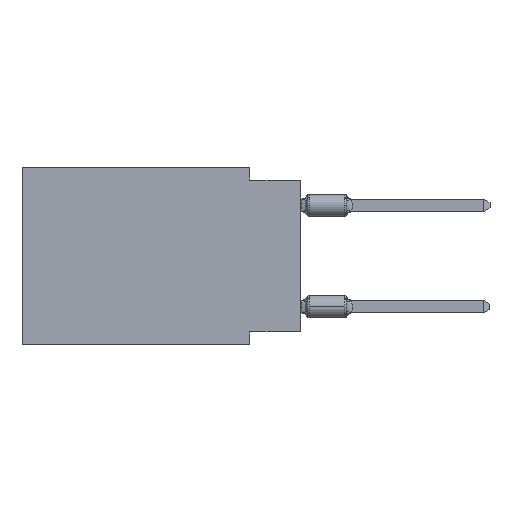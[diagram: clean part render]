
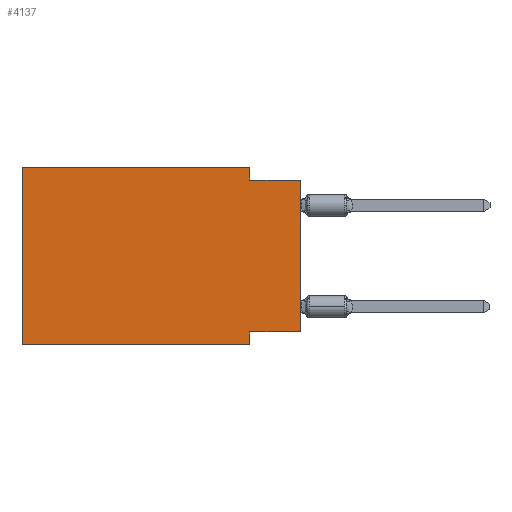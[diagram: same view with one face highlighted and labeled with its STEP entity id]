
A CAD part, left-side view. The second image highlights one B-rep face of the part: STEP entity #4137.
In plain terms, the highlighted planar face has unit normal (-1, 0, 0).
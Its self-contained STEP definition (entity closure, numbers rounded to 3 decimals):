
#180 = DIRECTION ( 'NONE',  ( 0., -1., 0. ) ) ;
#458 = CARTESIAN_POINT ( 'NONE',  ( 0., 2.54, -8.255 ) ) ;
#509 = LINE ( 'NONE', #15737, #996 ) ;
#527 = VERTEX_POINT ( 'NONE', #16872 ) ;
#996 = VECTOR ( 'NONE', #14540, 1000. ) ;
#1173 = ORIENTED_EDGE ( 'NONE', *, *, #3912, .F. ) ;
#1175 = FACE_OUTER_BOUND ( 'NONE', #7947, .T. ) ;
#1199 = EDGE_CURVE ( 'NONE', #1926, #527, #4851, .T. ) ;
#1754 = EDGE_CURVE ( 'NONE', #10161, #5200, #15205, .T. ) ;
#1926 = VERTEX_POINT ( 'NONE', #11672 ) ;
#2399 = DIRECTION ( 'NONE',  ( 0., 0., 1. ) ) ;
#2541 = VECTOR ( 'NONE', #3066, 1000. ) ;
#2584 = VECTOR ( 'NONE', #14781, 1000. ) ;
#2741 = DIRECTION ( 'NONE',  ( 1., 0., 0. ) ) ;
#3066 = DIRECTION ( 'NONE',  ( 0., 0., -1. ) ) ;
#3123 = DIRECTION ( 'NONE',  ( 0., 1., 0. ) ) ;
#3416 = AXIS2_PLACEMENT_3D ( 'NONE', #5539, #2741, #8231 ) ;
#3437 = EDGE_CURVE ( 'NONE', #12481, #14654, #7340, .T. ) ;
#3444 = CARTESIAN_POINT ( 'NONE',  ( 0., 13.97, 0. ) ) ;
#3635 = ORIENTED_EDGE ( 'NONE', *, *, #3437, .F. ) ;
#3912 = EDGE_CURVE ( 'NONE', #7679, #16184, #11952, .T. ) ;
#4137 = ADVANCED_FACE ( 'NONE', ( #1175 ), #9712, .F. ) ;
#4370 = VECTOR ( 'NONE', #180, 1000. ) ;
#4851 = LINE ( 'NONE', #3444, #2584 ) ;
#4991 = CARTESIAN_POINT ( 'NONE',  ( 0., 0., -8.255 ) ) ;
#5200 = VERTEX_POINT ( 'NONE', #7617 ) ;
#5261 = ORIENTED_EDGE ( 'NONE', *, *, #1754, .T. ) ;
#5475 = DIRECTION ( 'NONE',  ( 0., -1., 0. ) ) ;
#5486 = VECTOR ( 'NONE', #17693, 1000. ) ;
#5539 = CARTESIAN_POINT ( 'NONE',  ( 0., 13.97, 0. ) ) ;
#6037 = CARTESIAN_POINT ( 'NONE',  ( 0., 13.97, 0. ) ) ;
#6920 = ORIENTED_EDGE ( 'NONE', *, *, #1199, .F. ) ;
#7244 = LINE ( 'NONE', #6037, #4370 ) ;
#7340 = LINE ( 'NONE', #17441, #2541 ) ;
#7617 = CARTESIAN_POINT ( 'NONE',  ( 0., 0., -0.635 ) ) ;
#7679 = VERTEX_POINT ( 'NONE', #14982 ) ;
#7947 = EDGE_LOOP ( 'NONE', ( #5261, #17513, #1173, #12403, #6920, #12922, #3635, #14546 ) ) ;
#8231 = DIRECTION ( 'NONE',  ( 0., 0., -1. ) ) ;
#9651 = CARTESIAN_POINT ( 'NONE',  ( 0., 0., -0.635 ) ) ;
#9712 = PLANE ( 'NONE',  #3416 ) ;
#10161 = VERTEX_POINT ( 'NONE', #16124 ) ;
#10268 = LINE ( 'NONE', #4991, #15019 ) ;
#11464 = EDGE_CURVE ( 'NONE', #1926, #14654, #509, .T. ) ;
#11672 = CARTESIAN_POINT ( 'NONE',  ( 0., 13.97, -8.89 ) ) ;
#11952 = LINE ( 'NONE', #14836, #5486 ) ;
#12030 = CARTESIAN_POINT ( 'NONE',  ( 0., 2.54, -8.89 ) ) ;
#12244 = CARTESIAN_POINT ( 'NONE',  ( 0., 0., 0. ) ) ;
#12403 = ORIENTED_EDGE ( 'NONE', *, *, #18184, .F. ) ;
#12481 = VERTEX_POINT ( 'NONE', #458 ) ;
#12504 = EDGE_CURVE ( 'NONE', #16184, #5200, #17448, .T. ) ;
#12922 = ORIENTED_EDGE ( 'NONE', *, *, #11464, .T. ) ;
#13039 = CARTESIAN_POINT ( 'NONE',  ( 0., 2.54, -0.635 ) ) ;
#13814 = VECTOR ( 'NONE', #5475, 1000. ) ;
#14540 = DIRECTION ( 'NONE',  ( 0., -1., 0. ) ) ;
#14546 = ORIENTED_EDGE ( 'NONE', *, *, #15736, .F. ) ;
#14654 = VERTEX_POINT ( 'NONE', #12030 ) ;
#14781 = DIRECTION ( 'NONE',  ( 0., 0., 1. ) ) ;
#14836 = CARTESIAN_POINT ( 'NONE',  ( 0., 2.54, 0. ) ) ;
#14982 = CARTESIAN_POINT ( 'NONE',  ( 0., 2.54, 0. ) ) ;
#15019 = VECTOR ( 'NONE', #3123, 1000. ) ;
#15205 = LINE ( 'NONE', #12244, #17113 ) ;
#15736 = EDGE_CURVE ( 'NONE', #10161, #12481, #10268, .T. ) ;
#15737 = CARTESIAN_POINT ( 'NONE',  ( 0., 13.97, -8.89 ) ) ;
#16124 = CARTESIAN_POINT ( 'NONE',  ( 0., 0., -8.255 ) ) ;
#16184 = VERTEX_POINT ( 'NONE', #13039 ) ;
#16872 = CARTESIAN_POINT ( 'NONE',  ( 0., 13.97, 0. ) ) ;
#17113 = VECTOR ( 'NONE', #2399, 1000. ) ;
#17441 = CARTESIAN_POINT ( 'NONE',  ( 0., 2.54, -8.89 ) ) ;
#17448 = LINE ( 'NONE', #9651, #13814 ) ;
#17513 = ORIENTED_EDGE ( 'NONE', *, *, #12504, .F. ) ;
#17693 = DIRECTION ( 'NONE',  ( 0., 0., -1. ) ) ;
#18184 = EDGE_CURVE ( 'NONE', #527, #7679, #7244, .T. ) ;
